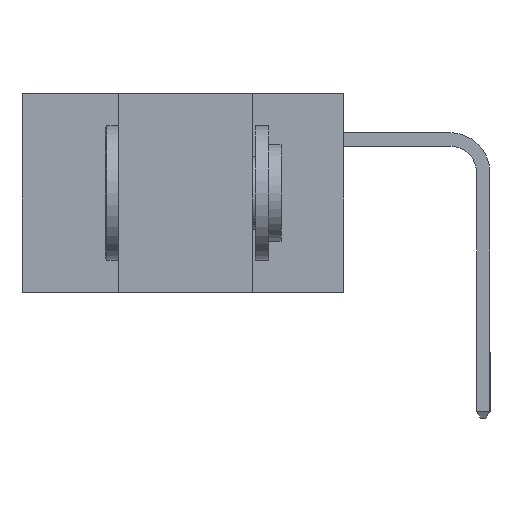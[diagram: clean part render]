
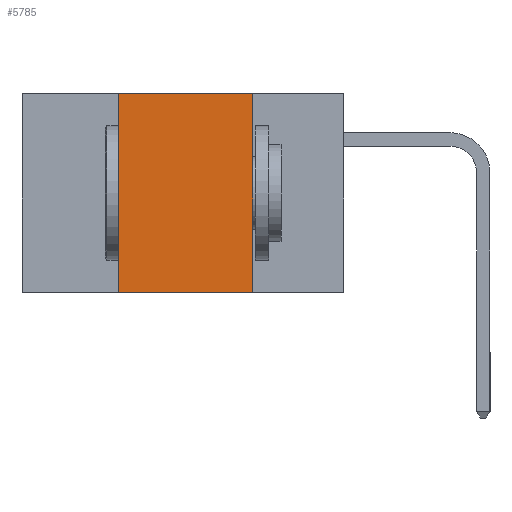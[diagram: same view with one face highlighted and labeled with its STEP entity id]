
A CAD part, left-side view. The second image highlights one B-rep face of the part: STEP entity #5785.
In plain terms, the highlighted planar face has unit normal (-1, 0, 0).
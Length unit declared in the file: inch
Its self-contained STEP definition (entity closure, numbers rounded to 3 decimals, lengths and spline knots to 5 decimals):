
#541 = CARTESIAN_POINT ( 'NONE',  ( 0., 0.6, -0.37 ) ) ;
#636 = VECTOR ( 'NONE', #9757, 39.37008 ) ;
#1372 = DIRECTION ( 'NONE',  ( 1., 0., 0. ) ) ;
#1659 = VERTEX_POINT ( 'NONE', #11342 ) ;
#1853 = VERTEX_POINT ( 'NONE', #11066 ) ;
#2123 = CARTESIAN_POINT ( 'NONE',  ( 0., 0.17, 0. ) ) ;
#2133 = VERTEX_POINT ( 'NONE', #2592 ) ;
#2436 = CARTESIAN_POINT ( 'NONE',  ( 0., 0.17, 0. ) ) ;
#2557 = DIRECTION ( 'NONE',  ( 0., 0., -1. ) ) ;
#2592 = CARTESIAN_POINT ( 'NONE',  ( 0., 0.42, 0. ) ) ;
#3407 = EDGE_CURVE ( 'NONE', #1659, #2133, #8807, .T. ) ;
#3916 = LINE ( 'NONE', #541, #14454 ) ;
#4121 = ORIENTED_EDGE ( 'NONE', *, *, #8955, .F. ) ;
#5785 = ADVANCED_FACE ( 'NONE', ( #6203 ), #6120, .F. ) ;
#6120 = PLANE ( 'NONE',  #7013 ) ;
#6203 = FACE_OUTER_BOUND ( 'NONE', #15865, .T. ) ;
#7013 = AXIS2_PLACEMENT_3D ( 'NONE', #13715, #1372, #2557 ) ;
#8031 = LINE ( 'NONE', #10714, #13900 ) ;
#8521 = VERTEX_POINT ( 'NONE', #2436 ) ;
#8807 = LINE ( 'NONE', #13568, #636 ) ;
#8955 = EDGE_CURVE ( 'NONE', #2133, #8521, #8031, .T. ) ;
#9693 = DIRECTION ( 'NONE',  ( 0., 0., -1. ) ) ;
#9757 = DIRECTION ( 'NONE',  ( 0., 0., 1. ) ) ;
#10651 = LINE ( 'NONE', #2123, #13545 ) ;
#10714 = CARTESIAN_POINT ( 'NONE',  ( 0., 0.6, 0. ) ) ;
#11035 = ORIENTED_EDGE ( 'NONE', *, *, #12875, .T. ) ;
#11066 = CARTESIAN_POINT ( 'NONE',  ( 0., 0.17, -0.37 ) ) ;
#11151 = EDGE_CURVE ( 'NONE', #8521, #1853, #10651, .T. ) ;
#11342 = CARTESIAN_POINT ( 'NONE',  ( 0., 0.42, -0.37 ) ) ;
#11921 = DIRECTION ( 'NONE',  ( 0., -1., 0. ) ) ;
#12019 = ORIENTED_EDGE ( 'NONE', *, *, #11151, .F. ) ;
#12875 = EDGE_CURVE ( 'NONE', #1659, #1853, #3916, .T. ) ;
#13545 = VECTOR ( 'NONE', #9693, 39.37008 ) ;
#13568 = CARTESIAN_POINT ( 'NONE',  ( 0., 0.42, 0. ) ) ;
#13715 = CARTESIAN_POINT ( 'NONE',  ( 0., 0.6, 0. ) ) ;
#13900 = VECTOR ( 'NONE', #11921, 39.37008 ) ;
#14180 = ORIENTED_EDGE ( 'NONE', *, *, #3407, .F. ) ;
#14274 = DIRECTION ( 'NONE',  ( 0., -1., 0. ) ) ;
#14454 = VECTOR ( 'NONE', #14274, 39.37008 ) ;
#15865 = EDGE_LOOP ( 'NONE', ( #12019, #4121, #14180, #11035 ) ) ;
